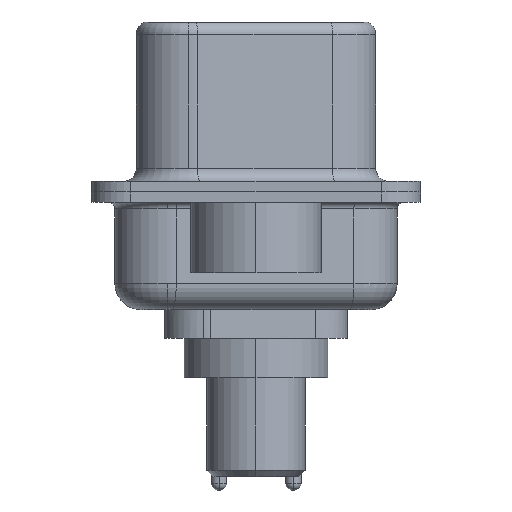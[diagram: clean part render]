
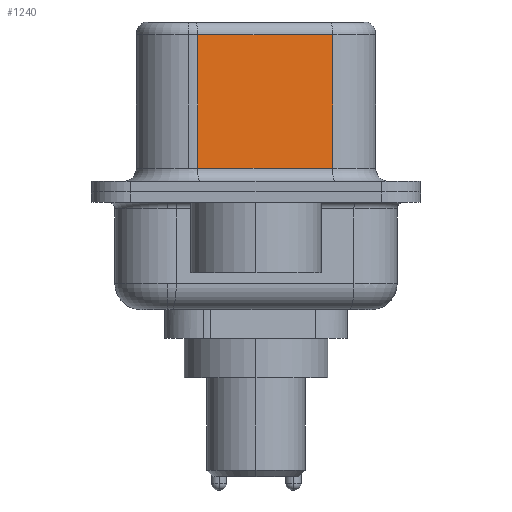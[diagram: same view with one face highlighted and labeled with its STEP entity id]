
A CAD part, left-side view. The second image highlights one B-rep face of the part: STEP entity #1240.
In plain terms, the highlighted planar face has unit normal (-0.985, -0.174, 0).
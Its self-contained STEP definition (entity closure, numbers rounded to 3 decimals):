
#332 = EDGE_CURVE ( 'NONE', #17124, #10668, #1272, .T. ) ;
#501 = DIRECTION ( 'NONE',  ( -0.174, 0.985, 0. ) ) ;
#582 = VERTEX_POINT ( 'NONE', #6878 ) ;
#709 = ORIENTED_EDGE ( 'NONE', *, *, #15964, .F. ) ;
#1240 = ADVANCED_FACE ( 'NONE', ( #9131 ), #14397, .F. ) ;
#1272 = LINE ( 'NONE', #13800, #8764 ) ;
#1437 = VECTOR ( 'NONE', #5764, 1000. ) ;
#1861 = LINE ( 'NONE', #2936, #1437 ) ;
#1974 = DIRECTION ( 'NONE',  ( 0.985, 0.174, 0. ) ) ;
#2133 = LINE ( 'NONE', #7692, #16803 ) ;
#2608 = VECTOR ( 'NONE', #12261, 1000. ) ;
#2936 = CARTESIAN_POINT ( 'NONE',  ( 4.565, -2.927, 6.02 ) ) ;
#4061 = CARTESIAN_POINT ( 'NONE',  ( 4.565, -2.927, 6.02 ) ) ;
#5063 = DIRECTION ( 'NONE',  ( 0.174, -0.985, 0. ) ) ;
#5764 = DIRECTION ( 'NONE',  ( -0.174, 0.985, 0. ) ) ;
#6878 = CARTESIAN_POINT ( 'NONE',  ( 4.565, -2.927, 0.9 ) ) ;
#7587 = EDGE_LOOP ( 'NONE', ( #709, #8376, #9182, #11261 ) ) ;
#7692 = CARTESIAN_POINT ( 'NONE',  ( 4.565, -2.927, 0.9 ) ) ;
#8376 = ORIENTED_EDGE ( 'NONE', *, *, #12416, .T. ) ;
#8764 = VECTOR ( 'NONE', #13888, 1000. ) ;
#9037 = CARTESIAN_POINT ( 'NONE',  ( 3.655, 2.233, 0.9 ) ) ;
#9131 = FACE_OUTER_BOUND ( 'NONE', #7587, .T. ) ;
#9182 = ORIENTED_EDGE ( 'NONE', *, *, #332, .T. ) ;
#10578 = CARTESIAN_POINT ( 'NONE',  ( 3.655, 2.233, 6.02 ) ) ;
#10668 = VERTEX_POINT ( 'NONE', #9037 ) ;
#10845 = CARTESIAN_POINT ( 'NONE',  ( 4.565, -2.927, 6.52 ) ) ;
#11261 = ORIENTED_EDGE ( 'NONE', *, *, #16421, .T. ) ;
#12261 = DIRECTION ( 'NONE',  ( 0., 0., -1. ) ) ;
#12416 = EDGE_CURVE ( 'NONE', #16057, #17124, #1861, .T. ) ;
#13474 = CARTESIAN_POINT ( 'NONE',  ( 4.565, -2.927, 6.52 ) ) ;
#13800 = CARTESIAN_POINT ( 'NONE',  ( 3.655, 2.233, 6.52 ) ) ;
#13888 = DIRECTION ( 'NONE',  ( 0., 0., -1. ) ) ;
#14397 = PLANE ( 'NONE',  #15523 ) ;
#15523 = AXIS2_PLACEMENT_3D ( 'NONE', #13474, #1974, #501 ) ;
#15964 = EDGE_CURVE ( 'NONE', #16057, #582, #16819, .T. ) ;
#16057 = VERTEX_POINT ( 'NONE', #4061 ) ;
#16421 = EDGE_CURVE ( 'NONE', #10668, #582, #2133, .T. ) ;
#16803 = VECTOR ( 'NONE', #5063, 1000. ) ;
#16819 = LINE ( 'NONE', #10845, #2608 ) ;
#17124 = VERTEX_POINT ( 'NONE', #10578 ) ;
